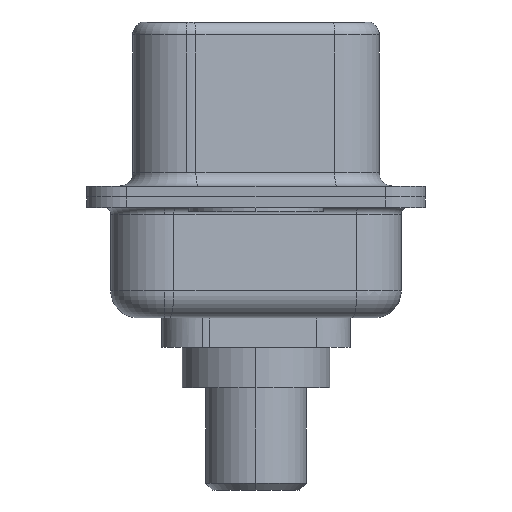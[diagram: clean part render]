
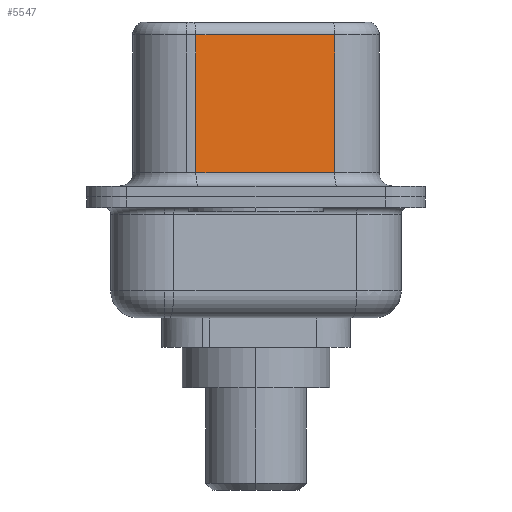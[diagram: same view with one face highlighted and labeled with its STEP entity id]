
A CAD part, left-side view. The second image highlights one B-rep face of the part: STEP entity #5547.
In plain terms, the highlighted planar face has unit normal (-0.985, -0.174, 0).
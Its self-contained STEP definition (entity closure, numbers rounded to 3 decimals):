
#547 = VECTOR ( 'NONE', #6221, 1000. ) ;
#1262 = LINE ( 'NONE', #3714, #6343 ) ;
#1375 = EDGE_LOOP ( 'NONE', ( #8726, #5831, #6961, #6739 ) ) ;
#1999 = DIRECTION ( 'NONE',  ( 0.985, 0.174, 0. ) ) ;
#2304 = CARTESIAN_POINT ( 'NONE',  ( 4.58, -2.927, 0.9 ) ) ;
#2917 = FACE_OUTER_BOUND ( 'NONE', #1375, .T. ) ;
#2985 = EDGE_CURVE ( 'NONE', #11279, #4344, #9290, .T. ) ;
#3322 = EDGE_CURVE ( 'NONE', #11990, #4344, #12305, .T. ) ;
#3714 = CARTESIAN_POINT ( 'NONE',  ( 3.67, 2.233, 6.52 ) ) ;
#3954 = AXIS2_PLACEMENT_3D ( 'NONE', #9850, #1999, #9568 ) ;
#4294 = EDGE_CURVE ( 'NONE', #4565, #11279, #1262, .T. ) ;
#4344 = VERTEX_POINT ( 'NONE', #7818 ) ;
#4421 = VECTOR ( 'NONE', #10154, 1000. ) ;
#4517 = CARTESIAN_POINT ( 'NONE',  ( 4.58, -2.927, 6.52 ) ) ;
#4565 = VERTEX_POINT ( 'NONE', #11207 ) ;
#5547 = ADVANCED_FACE ( 'NONE', ( #2917 ), #12114, .F. ) ;
#5831 = ORIENTED_EDGE ( 'NONE', *, *, #9388, .T. ) ;
#6001 = CARTESIAN_POINT ( 'NONE',  ( 4.58, -2.927, 6.02 ) ) ;
#6197 = CARTESIAN_POINT ( 'NONE',  ( 4.58, -2.927, 6.02 ) ) ;
#6221 = DIRECTION ( 'NONE',  ( -0.174, 0.985, 0. ) ) ;
#6343 = VECTOR ( 'NONE', #8929, 1000. ) ;
#6739 = ORIENTED_EDGE ( 'NONE', *, *, #2985, .T. ) ;
#6961 = ORIENTED_EDGE ( 'NONE', *, *, #4294, .T. ) ;
#7818 = CARTESIAN_POINT ( 'NONE',  ( 4.58, -2.927, 0.9 ) ) ;
#8726 = ORIENTED_EDGE ( 'NONE', *, *, #3322, .F. ) ;
#8929 = DIRECTION ( 'NONE',  ( 0., 0., -1. ) ) ;
#9290 = LINE ( 'NONE', #2304, #4421 ) ;
#9388 = EDGE_CURVE ( 'NONE', #11990, #4565, #11043, .T. ) ;
#9550 = CARTESIAN_POINT ( 'NONE',  ( 3.67, 2.233, 0.9 ) ) ;
#9568 = DIRECTION ( 'NONE',  ( -0.174, 0.985, 0. ) ) ;
#9850 = CARTESIAN_POINT ( 'NONE',  ( 4.58, -2.927, 6.52 ) ) ;
#9852 = VECTOR ( 'NONE', #10816, 1000. ) ;
#10154 = DIRECTION ( 'NONE',  ( 0.174, -0.985, 0. ) ) ;
#10816 = DIRECTION ( 'NONE',  ( 0., 0., -1. ) ) ;
#11043 = LINE ( 'NONE', #6001, #547 ) ;
#11207 = CARTESIAN_POINT ( 'NONE',  ( 3.67, 2.233, 6.02 ) ) ;
#11279 = VERTEX_POINT ( 'NONE', #9550 ) ;
#11990 = VERTEX_POINT ( 'NONE', #6197 ) ;
#12114 = PLANE ( 'NONE',  #3954 ) ;
#12305 = LINE ( 'NONE', #4517, #9852 ) ;
